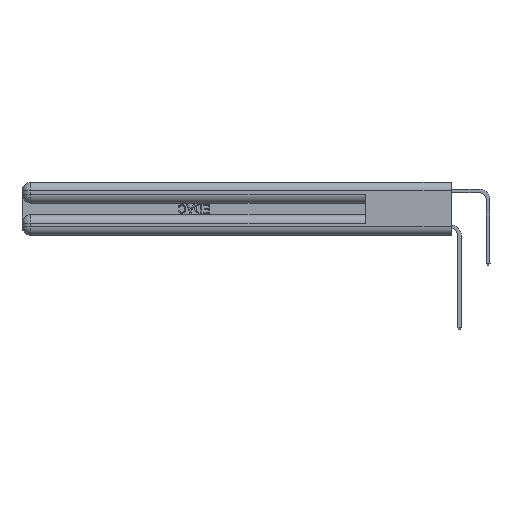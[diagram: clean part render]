
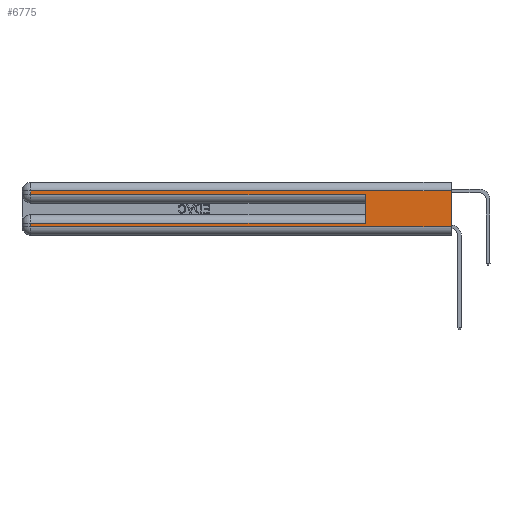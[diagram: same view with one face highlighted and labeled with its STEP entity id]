
A CAD part, left-side view. The second image highlights one B-rep face of the part: STEP entity #6775.
In plain terms, the highlighted planar face has unit normal (-1, 0, 0).
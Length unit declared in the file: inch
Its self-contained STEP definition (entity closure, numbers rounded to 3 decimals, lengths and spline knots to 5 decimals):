
#474 = ORIENTED_EDGE ( 'NONE', *, *, #29205, .T. ) ;
#717 = VECTOR ( 'NONE', #1728, 39.37008 ) ;
#778 = VECTOR ( 'NONE', #19398, 39.37008 ) ;
#1128 = DIRECTION ( 'NONE',  ( 1., 0., 0. ) ) ;
#1728 = DIRECTION ( 'NONE',  ( 0., 0., -1. ) ) ;
#2124 = DIRECTION ( 'NONE',  ( 0., 0., 1. ) ) ;
#2302 = ORIENTED_EDGE ( 'NONE', *, *, #12785, .F. ) ;
#3553 = EDGE_CURVE ( 'NONE', #16982, #21457, #4945, .T. ) ;
#3889 = ORIENTED_EDGE ( 'NONE', *, *, #26253, .T. ) ;
#3985 = CARTESIAN_POINT ( 'NONE',  ( 0., 2.94, 0.37 ) ) ;
#4517 = VERTEX_POINT ( 'NONE', #23572 ) ;
#4945 = LINE ( 'NONE', #16299, #21200 ) ;
#5226 = EDGE_CURVE ( 'NONE', #4517, #26185, #30785, .T. ) ;
#6320 = VECTOR ( 'NONE', #23545, 39.37008 ) ;
#6495 = VECTOR ( 'NONE', #19128, 39.37008 ) ;
#6657 = CARTESIAN_POINT ( 'NONE',  ( 0., 0., 0.37 ) ) ;
#6775 = ADVANCED_FACE ( 'NONE', ( #18190 ), #13030, .F. ) ;
#7804 = LINE ( 'NONE', #6657, #6320 ) ;
#8443 = LINE ( 'NONE', #16373, #22109 ) ;
#9111 = CARTESIAN_POINT ( 'NONE',  ( 0., 2.94, 0.31 ) ) ;
#9998 = CARTESIAN_POINT ( 'NONE',  ( 0., 0., 0.31 ) ) ;
#10173 = DIRECTION ( 'NONE',  ( 0., -1., 0. ) ) ;
#10505 = CARTESIAN_POINT ( 'NONE',  ( 0., 0., 0.37 ) ) ;
#10928 = DIRECTION ( 'NONE',  ( 0., 0., -1. ) ) ;
#10953 = CARTESIAN_POINT ( 'NONE',  ( 0., 0.6, 0.085 ) ) ;
#11188 = ORIENTED_EDGE ( 'NONE', *, *, #27034, .F. ) ;
#11776 = CARTESIAN_POINT ( 'NONE',  ( 0., 2.94, 0.37 ) ) ;
#12785 = EDGE_CURVE ( 'NONE', #16982, #24401, #7804, .T. ) ;
#13030 = PLANE ( 'NONE',  #25943 ) ;
#13971 = CARTESIAN_POINT ( 'NONE',  ( 0., 2.94, 0.06 ) ) ;
#15631 = VECTOR ( 'NONE', #10173, 39.37008 ) ;
#16299 = CARTESIAN_POINT ( 'NONE',  ( 0., 0., 0.31 ) ) ;
#16373 = CARTESIAN_POINT ( 'NONE',  ( 0., 0.6, 0.145 ) ) ;
#16589 = CARTESIAN_POINT ( 'NONE',  ( 0., 0., 0.085 ) ) ;
#16982 = VERTEX_POINT ( 'NONE', #9998 ) ;
#18190 = FACE_OUTER_BOUND ( 'NONE', #29785, .T. ) ;
#18210 = ORIENTED_EDGE ( 'NONE', *, *, #30975, .T. ) ;
#18834 = DIRECTION ( 'NONE',  ( 0., 1., 0. ) ) ;
#19128 = DIRECTION ( 'NONE',  ( 0., 1., 0. ) ) ;
#19398 = DIRECTION ( 'NONE',  ( 0., 0., -1. ) ) ;
#20654 = CARTESIAN_POINT ( 'NONE',  ( 0., 0.6, 0.285 ) ) ;
#20711 = VERTEX_POINT ( 'NONE', #28037 ) ;
#21200 = VECTOR ( 'NONE', #18834, 39.37008 ) ;
#21457 = VERTEX_POINT ( 'NONE', #9111 ) ;
#22109 = VECTOR ( 'NONE', #2124, 39.37008 ) ;
#22237 = CARTESIAN_POINT ( 'NONE',  ( 0., 0., 0.06 ) ) ;
#22686 = LINE ( 'NONE', #11776, #778 ) ;
#23297 = VECTOR ( 'NONE', #27832, 39.37008 ) ;
#23328 = VERTEX_POINT ( 'NONE', #10953 ) ;
#23545 = DIRECTION ( 'NONE',  ( 0., 0., -1. ) ) ;
#23572 = CARTESIAN_POINT ( 'NONE',  ( 0., 2.94, 0.285 ) ) ;
#24067 = LINE ( 'NONE', #30467, #23297 ) ;
#24401 = VERTEX_POINT ( 'NONE', #22237 ) ;
#25118 = ORIENTED_EDGE ( 'NONE', *, *, #5226, .T. ) ;
#25943 = AXIS2_PLACEMENT_3D ( 'NONE', #10505, #1128, #10928 ) ;
#26185 = VERTEX_POINT ( 'NONE', #20654 ) ;
#26253 = EDGE_CURVE ( 'NONE', #27907, #24401, #24067, .T. ) ;
#26518 = LINE ( 'NONE', #16589, #6495 ) ;
#27034 = EDGE_CURVE ( 'NONE', #23328, #26185, #8443, .T. ) ;
#27199 = CARTESIAN_POINT ( 'NONE',  ( 0., 0., 0.285 ) ) ;
#27832 = DIRECTION ( 'NONE',  ( 0., -1., 0. ) ) ;
#27907 = VERTEX_POINT ( 'NONE', #13971 ) ;
#28037 = CARTESIAN_POINT ( 'NONE',  ( 0., 2.94, 0.085 ) ) ;
#28580 = ORIENTED_EDGE ( 'NONE', *, *, #28656, .T. ) ;
#28656 = EDGE_CURVE ( 'NONE', #23328, #20711, #26518, .T. ) ;
#29059 = LINE ( 'NONE', #3985, #717 ) ;
#29205 = EDGE_CURVE ( 'NONE', #20711, #27907, #22686, .T. ) ;
#29785 = EDGE_LOOP ( 'NONE', ( #2302, #31059, #18210, #25118, #11188, #28580, #474, #3889 ) ) ;
#30467 = CARTESIAN_POINT ( 'NONE',  ( 0., 0., 0.06 ) ) ;
#30785 = LINE ( 'NONE', #27199, #15631 ) ;
#30975 = EDGE_CURVE ( 'NONE', #21457, #4517, #29059, .T. ) ;
#31059 = ORIENTED_EDGE ( 'NONE', *, *, #3553, .T. ) ;
